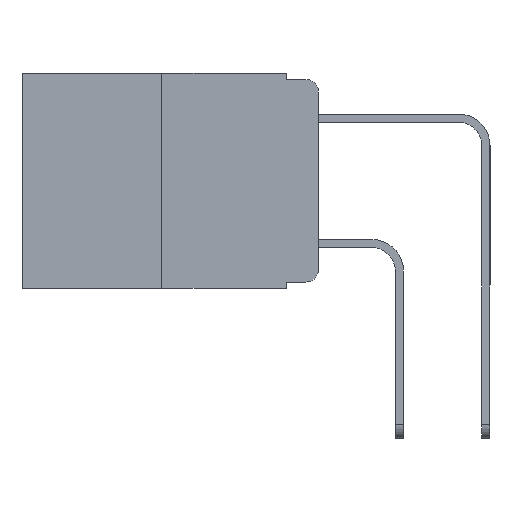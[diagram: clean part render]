
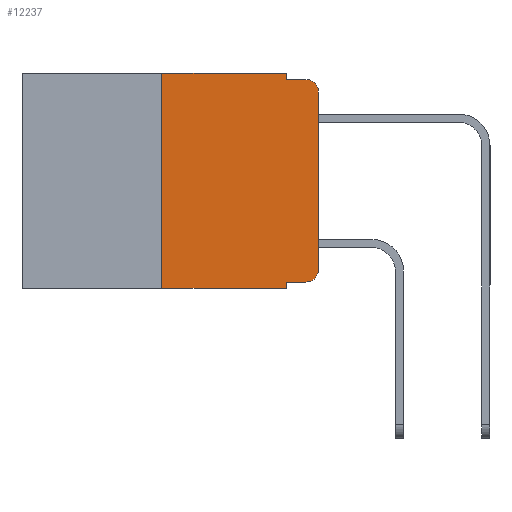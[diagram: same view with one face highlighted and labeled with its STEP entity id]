
A CAD part, left-side view. The second image highlights one B-rep face of the part: STEP entity #12237.
In plain terms, the highlighted planar face has unit normal (-1, 0, 0).
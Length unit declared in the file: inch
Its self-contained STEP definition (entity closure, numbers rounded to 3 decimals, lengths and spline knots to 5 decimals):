
#44 = VECTOR ( 'NONE', #2541, 39.37008 ) ;
#96 = CARTESIAN_POINT ( 'NONE',  ( 0., 0., -0.03 ) ) ;
#130 = EDGE_CURVE ( 'NONE', #8128, #7294, #12138, .T. ) ;
#724 = VECTOR ( 'NONE', #6568, 39.37008 ) ;
#1372 = FACE_OUTER_BOUND ( 'NONE', #4489, .T. ) ;
#1571 = ORIENTED_EDGE ( 'NONE', *, *, #9997, .F. ) ;
#1814 = EDGE_CURVE ( 'NONE', #6056, #8128, #11172, .T. ) ;
#2051 = CARTESIAN_POINT ( 'NONE',  ( 0., 0.25, 0. ) ) ;
#2068 = DIRECTION ( 'NONE',  ( -1., 0., 0. ) ) ;
#2347 = CARTESIAN_POINT ( 'NONE',  ( 0., 0.25, -0.343 ) ) ;
#2541 = DIRECTION ( 'NONE',  ( 0., -1., 0. ) ) ;
#2561 = ORIENTED_EDGE ( 'NONE', *, *, #4572, .T. ) ;
#2632 = VERTEX_POINT ( 'NONE', #11903 ) ;
#2961 = LINE ( 'NONE', #13478, #11851 ) ;
#3055 = DIRECTION ( 'NONE',  ( -1., 0., 0. ) ) ;
#3195 = ORIENTED_EDGE ( 'NONE', *, *, #14511, .F. ) ;
#3531 = ORIENTED_EDGE ( 'NONE', *, *, #11492, .F. ) ;
#3684 = CARTESIAN_POINT ( 'NONE',  ( 0., 0.051, -0.333 ) ) ;
#4489 = EDGE_LOOP ( 'NONE', ( #14910, #8032, #3195, #5280, #6764, #3531, #2561, #1571, #5688, #5160 ) ) ;
#4572 = EDGE_CURVE ( 'NONE', #12793, #10159, #13932, .T. ) ;
#4602 = CARTESIAN_POINT ( 'NONE',  ( 0., 0., -0.313 ) ) ;
#4737 = CARTESIAN_POINT ( 'NONE',  ( 0., 0.051, -0.01 ) ) ;
#4749 = AXIS2_PLACEMENT_3D ( 'NONE', #9149, #2068, #10278 ) ;
#4986 = CARTESIAN_POINT ( 'NONE',  ( 0., 0.473, 0. ) ) ;
#5160 = ORIENTED_EDGE ( 'NONE', *, *, #8492, .T. ) ;
#5188 = CARTESIAN_POINT ( 'NONE',  ( 0., 0.051, -0.333 ) ) ;
#5280 = ORIENTED_EDGE ( 'NONE', *, *, #13758, .F. ) ;
#5309 = LINE ( 'NONE', #4737, #14058 ) ;
#5688 = ORIENTED_EDGE ( 'NONE', *, *, #9260, .T. ) ;
#5904 = VECTOR ( 'NONE', #10265, 39.37008 ) ;
#6056 = VERTEX_POINT ( 'NONE', #4602 ) ;
#6174 = DIRECTION ( 'NONE',  ( 0., -1., 0. ) ) ;
#6491 = LINE ( 'NONE', #3684, #44 ) ;
#6568 = DIRECTION ( 'NONE',  ( 0., 0., -1. ) ) ;
#6764 = ORIENTED_EDGE ( 'NONE', *, *, #10957, .F. ) ;
#6965 = AXIS2_PLACEMENT_3D ( 'NONE', #10500, #13874, #7098 ) ;
#7057 = VERTEX_POINT ( 'NONE', #5188 ) ;
#7098 = DIRECTION ( 'NONE',  ( 0., 0., -1. ) ) ;
#7294 = VERTEX_POINT ( 'NONE', #10255 ) ;
#7960 = CARTESIAN_POINT ( 'NONE',  ( 0., 0.473, -0.343 ) ) ;
#7976 = DIRECTION ( 'NONE',  ( 0., 0., -1. ) ) ;
#8032 = ORIENTED_EDGE ( 'NONE', *, *, #130, .T. ) ;
#8128 = VERTEX_POINT ( 'NONE', #96 ) ;
#8163 = CARTESIAN_POINT ( 'NONE',  ( 0., 0.051, -0.343 ) ) ;
#8198 = VECTOR ( 'NONE', #12873, 39.37008 ) ;
#8213 = CARTESIAN_POINT ( 'NONE',  ( 0., 0.02, -0.333 ) ) ;
#8223 = PLANE ( 'NONE',  #6965 ) ;
#8492 = EDGE_CURVE ( 'NONE', #12744, #6056, #11532, .T. ) ;
#8996 = LINE ( 'NONE', #2051, #5904 ) ;
#9149 = CARTESIAN_POINT ( 'NONE',  ( 0., 0.02, -0.313 ) ) ;
#9260 = EDGE_CURVE ( 'NONE', #7057, #12744, #6491, .T. ) ;
#9281 = VERTEX_POINT ( 'NONE', #12948 ) ;
#9422 = CARTESIAN_POINT ( 'NONE',  ( 0., 0.051, -0.01 ) ) ;
#9997 = EDGE_CURVE ( 'NONE', #7057, #10159, #2961, .T. ) ;
#10159 = VERTEX_POINT ( 'NONE', #8163 ) ;
#10255 = CARTESIAN_POINT ( 'NONE',  ( 0., 0.02, -0.01 ) ) ;
#10265 = DIRECTION ( 'NONE',  ( 0., 0., 1. ) ) ;
#10278 = DIRECTION ( 'NONE',  ( 0., 0., -1. ) ) ;
#10500 = CARTESIAN_POINT ( 'NONE',  ( 0., 0.473, 0. ) ) ;
#10957 = EDGE_CURVE ( 'NONE', #2632, #9281, #12712, .T. ) ;
#11172 = LINE ( 'NONE', #11451, #8198 ) ;
#11187 = CARTESIAN_POINT ( 'NONE',  ( 0., 0.02, -0.03 ) ) ;
#11451 = CARTESIAN_POINT ( 'NONE',  ( 0., 0., 0. ) ) ;
#11492 = EDGE_CURVE ( 'NONE', #12793, #2632, #8996, .T. ) ;
#11532 = CIRCLE ( 'NONE', #4749, 0.02 ) ;
#11735 = AXIS2_PLACEMENT_3D ( 'NONE', #11187, #3055, #7976 ) ;
#11851 = VECTOR ( 'NONE', #14608, 39.37008 ) ;
#11903 = CARTESIAN_POINT ( 'NONE',  ( 0., 0.25, 0. ) ) ;
#12138 = CIRCLE ( 'NONE', #11735, 0.02 ) ;
#12237 = ADVANCED_FACE ( 'NONE', ( #1372 ), #8223, .F. ) ;
#12588 = DIRECTION ( 'NONE',  ( 0., -1., 0. ) ) ;
#12712 = LINE ( 'NONE', #4986, #13061 ) ;
#12744 = VERTEX_POINT ( 'NONE', #8213 ) ;
#12765 = DIRECTION ( 'NONE',  ( 0., -1., 0. ) ) ;
#12793 = VERTEX_POINT ( 'NONE', #2347 ) ;
#12873 = DIRECTION ( 'NONE',  ( 0., 0., 1. ) ) ;
#12948 = CARTESIAN_POINT ( 'NONE',  ( 0., 0.051, 0. ) ) ;
#13061 = VECTOR ( 'NONE', #6174, 39.37008 ) ;
#13388 = CARTESIAN_POINT ( 'NONE',  ( 0., 0.051, 0. ) ) ;
#13478 = CARTESIAN_POINT ( 'NONE',  ( 0., 0.051, 0. ) ) ;
#13503 = LINE ( 'NONE', #13388, #724 ) ;
#13584 = VECTOR ( 'NONE', #12588, 39.37008 ) ;
#13758 = EDGE_CURVE ( 'NONE', #9281, #15017, #13503, .T. ) ;
#13874 = DIRECTION ( 'NONE',  ( 1., 0., 0. ) ) ;
#13932 = LINE ( 'NONE', #7960, #13584 ) ;
#14058 = VECTOR ( 'NONE', #12765, 39.37008 ) ;
#14511 = EDGE_CURVE ( 'NONE', #15017, #7294, #5309, .T. ) ;
#14608 = DIRECTION ( 'NONE',  ( 0., 0., -1. ) ) ;
#14910 = ORIENTED_EDGE ( 'NONE', *, *, #1814, .T. ) ;
#15017 = VERTEX_POINT ( 'NONE', #9422 ) ;
